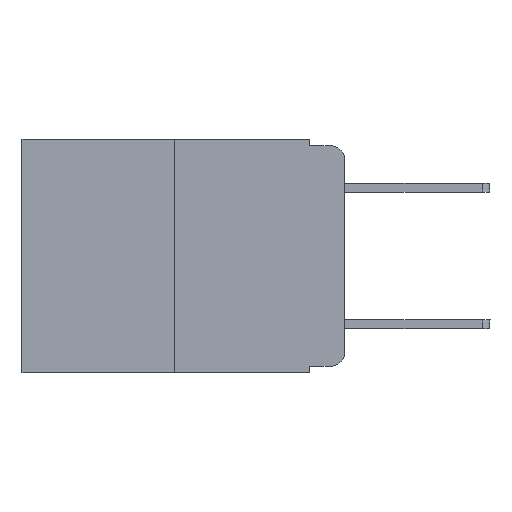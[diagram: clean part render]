
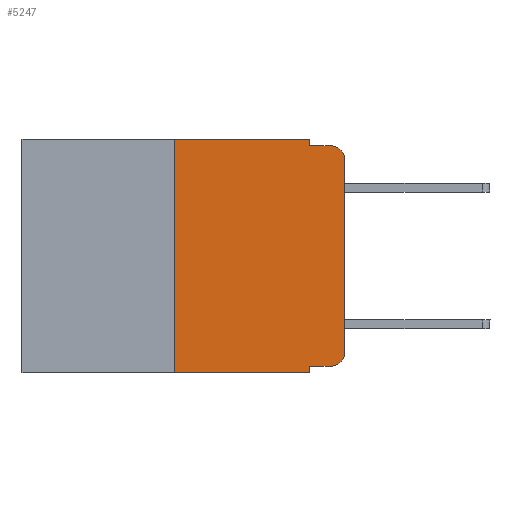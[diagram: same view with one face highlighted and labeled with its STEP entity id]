
A CAD part, left-side view. The second image highlights one B-rep face of the part: STEP entity #5247.
In plain terms, the highlighted planar face has unit normal (-1, 0, 0).
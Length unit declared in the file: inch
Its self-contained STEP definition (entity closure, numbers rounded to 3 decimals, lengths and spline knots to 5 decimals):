
#121 = CIRCLE ( 'NONE', #12135, 0.02 ) ;
#532 = VERTEX_POINT ( 'NONE', #5008 ) ;
#734 = CARTESIAN_POINT ( 'NONE',  ( 0., 0.25, -0.343 ) ) ;
#747 = EDGE_LOOP ( 'NONE', ( #3016, #857, #9560, #9270, #2226, #12046, #10466, #9740, #12698, #8888 ) ) ;
#857 = ORIENTED_EDGE ( 'NONE', *, *, #2621, .T. ) ;
#985 = LINE ( 'NONE', #6961, #12878 ) ;
#998 = VERTEX_POINT ( 'NONE', #12815 ) ;
#1244 = CARTESIAN_POINT ( 'NONE',  ( 0., 0.473, 0. ) ) ;
#1416 = VECTOR ( 'NONE', #4050, 39.37008 ) ;
#1495 = VERTEX_POINT ( 'NONE', #1812 ) ;
#1583 = CARTESIAN_POINT ( 'NONE',  ( 0., 0.473, 0. ) ) ;
#1644 = DIRECTION ( 'NONE',  ( 0., -1., 0. ) ) ;
#1777 = DIRECTION ( 'NONE',  ( 0., -1., 0. ) ) ;
#1812 = CARTESIAN_POINT ( 'NONE',  ( 0., 0.051, -0.01 ) ) ;
#1857 = VERTEX_POINT ( 'NONE', #4557 ) ;
#2162 = VERTEX_POINT ( 'NONE', #8677 ) ;
#2226 = ORIENTED_EDGE ( 'NONE', *, *, #7661, .F. ) ;
#2475 = CARTESIAN_POINT ( 'NONE',  ( 0., 0.051, 0. ) ) ;
#2528 = CARTESIAN_POINT ( 'NONE',  ( 0., 0.473, -0.343 ) ) ;
#2621 = EDGE_CURVE ( 'NONE', #2162, #1857, #121, .T. ) ;
#2859 = VECTOR ( 'NONE', #5487, 39.37008 ) ;
#3016 = ORIENTED_EDGE ( 'NONE', *, *, #6184, .T. ) ;
#3164 = DIRECTION ( 'NONE',  ( -1., 0., 0. ) ) ;
#3225 = VERTEX_POINT ( 'NONE', #734 ) ;
#3698 = LINE ( 'NONE', #5647, #5824 ) ;
#3855 = CARTESIAN_POINT ( 'NONE',  ( 0., 0.051, -0.01 ) ) ;
#3999 = VERTEX_POINT ( 'NONE', #11904 ) ;
#4050 = DIRECTION ( 'NONE',  ( 0., 0., 1. ) ) ;
#4243 = LINE ( 'NONE', #5067, #1416 ) ;
#4557 = CARTESIAN_POINT ( 'NONE',  ( 0., 0.02, -0.01 ) ) ;
#4628 = LINE ( 'NONE', #3855, #5687 ) ;
#4727 = EDGE_CURVE ( 'NONE', #7501, #3999, #12491, .T. ) ;
#5008 = CARTESIAN_POINT ( 'NONE',  ( 0., 0.051, -0.333 ) ) ;
#5067 = CARTESIAN_POINT ( 'NONE',  ( 0., 0.25, 0. ) ) ;
#5226 = LINE ( 'NONE', #1244, #2859 ) ;
#5247 = ADVANCED_FACE ( 'NONE', ( #5748 ), #6937, .F. ) ;
#5357 = LINE ( 'NONE', #2475, #5903 ) ;
#5487 = DIRECTION ( 'NONE',  ( 0., -1., 0. ) ) ;
#5647 = CARTESIAN_POINT ( 'NONE',  ( 0., 0., 0. ) ) ;
#5687 = VECTOR ( 'NONE', #1644, 39.37008 ) ;
#5748 = FACE_OUTER_BOUND ( 'NONE', #747, .T. ) ;
#5809 = DIRECTION ( 'NONE',  ( 1., 0., 0. ) ) ;
#5824 = VECTOR ( 'NONE', #12934, 39.37008 ) ;
#5903 = VECTOR ( 'NONE', #10706, 39.37008 ) ;
#6030 = DIRECTION ( 'NONE',  ( 0., -1., 0. ) ) ;
#6031 = CARTESIAN_POINT ( 'NONE',  ( 0., 0.02, -0.333 ) ) ;
#6184 = EDGE_CURVE ( 'NONE', #3999, #2162, #3698, .T. ) ;
#6329 = VERTEX_POINT ( 'NONE', #7044 ) ;
#6372 = DIRECTION ( 'NONE',  ( 0., 0., -1. ) ) ;
#6636 = DIRECTION ( 'NONE',  ( 0., 0., -1. ) ) ;
#6784 = EDGE_CURVE ( 'NONE', #532, #7501, #985, .T. ) ;
#6937 = PLANE ( 'NONE',  #8576 ) ;
#6961 = CARTESIAN_POINT ( 'NONE',  ( 0., 0.051, -0.333 ) ) ;
#7044 = CARTESIAN_POINT ( 'NONE',  ( 0., 0.051, 0. ) ) ;
#7234 = VERTEX_POINT ( 'NONE', #7439 ) ;
#7439 = CARTESIAN_POINT ( 'NONE',  ( 0., 0.051, -0.343 ) ) ;
#7501 = VERTEX_POINT ( 'NONE', #6031 ) ;
#7661 = EDGE_CURVE ( 'NONE', #998, #6329, #5226, .T. ) ;
#8429 = AXIS2_PLACEMENT_3D ( 'NONE', #8519, #3164, #6372 ) ;
#8514 = CARTESIAN_POINT ( 'NONE',  ( 0., 0.02, -0.03 ) ) ;
#8519 = CARTESIAN_POINT ( 'NONE',  ( 0., 0.02, -0.313 ) ) ;
#8576 = AXIS2_PLACEMENT_3D ( 'NONE', #1583, #5809, #12833 ) ;
#8677 = CARTESIAN_POINT ( 'NONE',  ( 0., 0., -0.03 ) ) ;
#8888 = ORIENTED_EDGE ( 'NONE', *, *, #4727, .T. ) ;
#8896 = VECTOR ( 'NONE', #1777, 39.37008 ) ;
#9270 = ORIENTED_EDGE ( 'NONE', *, *, #10245, .F. ) ;
#9377 = LINE ( 'NONE', #11447, #11891 ) ;
#9560 = ORIENTED_EDGE ( 'NONE', *, *, #10862, .F. ) ;
#9740 = ORIENTED_EDGE ( 'NONE', *, *, #11983, .F. ) ;
#9955 = LINE ( 'NONE', #2528, #8896 ) ;
#10245 = EDGE_CURVE ( 'NONE', #6329, #1495, #5357, .T. ) ;
#10466 = ORIENTED_EDGE ( 'NONE', *, *, #10740, .T. ) ;
#10706 = DIRECTION ( 'NONE',  ( 0., 0., -1. ) ) ;
#10740 = EDGE_CURVE ( 'NONE', #3225, #7234, #9955, .T. ) ;
#10834 = DIRECTION ( 'NONE',  ( 0., 0., -1. ) ) ;
#10862 = EDGE_CURVE ( 'NONE', #1495, #1857, #4628, .T. ) ;
#11447 = CARTESIAN_POINT ( 'NONE',  ( 0., 0.051, 0. ) ) ;
#11891 = VECTOR ( 'NONE', #10834, 39.37008 ) ;
#11904 = CARTESIAN_POINT ( 'NONE',  ( 0., 0., -0.313 ) ) ;
#11983 = EDGE_CURVE ( 'NONE', #532, #7234, #9377, .T. ) ;
#12046 = ORIENTED_EDGE ( 'NONE', *, *, #12687, .F. ) ;
#12135 = AXIS2_PLACEMENT_3D ( 'NONE', #8514, #12526, #6636 ) ;
#12491 = CIRCLE ( 'NONE', #8429, 0.02 ) ;
#12526 = DIRECTION ( 'NONE',  ( -1., 0., 0. ) ) ;
#12687 = EDGE_CURVE ( 'NONE', #3225, #998, #4243, .T. ) ;
#12698 = ORIENTED_EDGE ( 'NONE', *, *, #6784, .T. ) ;
#12815 = CARTESIAN_POINT ( 'NONE',  ( 0., 0.25, 0. ) ) ;
#12833 = DIRECTION ( 'NONE',  ( 0., 0., -1. ) ) ;
#12878 = VECTOR ( 'NONE', #6030, 39.37008 ) ;
#12934 = DIRECTION ( 'NONE',  ( 0., 0., 1. ) ) ;
